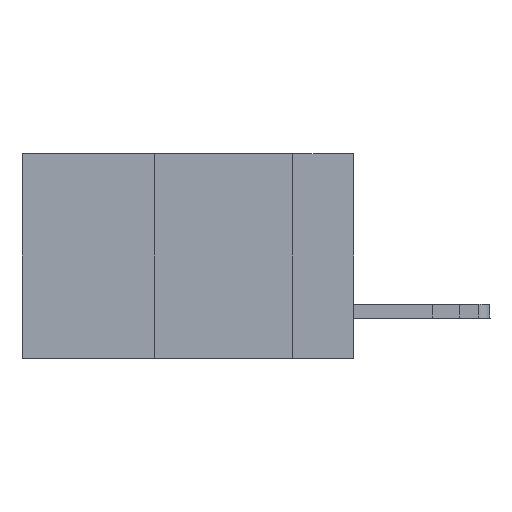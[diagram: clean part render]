
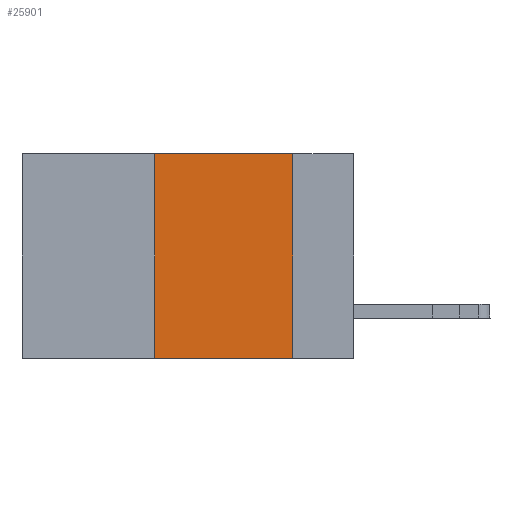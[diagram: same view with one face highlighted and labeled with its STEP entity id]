
A CAD part, left-side view. The second image highlights one B-rep face of the part: STEP entity #25901.
In plain terms, the highlighted planar face has unit normal (-1, 0, 0).
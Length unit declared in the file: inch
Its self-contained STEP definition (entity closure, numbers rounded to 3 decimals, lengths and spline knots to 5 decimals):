
#77 = EDGE_CURVE ( 'NONE', #2742, #160, #29321, .T. ) ;
#160 = VERTEX_POINT ( 'NONE', #16566 ) ;
#452 = VECTOR ( 'NONE', #12100, 39.37008 ) ;
#610 = ORIENTED_EDGE ( 'NONE', *, *, #16156, .F. ) ;
#1116 = CARTESIAN_POINT ( 'NONE',  ( 0., 0.36, -0.37 ) ) ;
#2742 = VERTEX_POINT ( 'NONE', #4361 ) ;
#3239 = VERTEX_POINT ( 'NONE', #1116 ) ;
#3292 = EDGE_LOOP ( 'NONE', ( #15563, #25573, #610, #14857 ) ) ;
#4238 = PLANE ( 'NONE',  #6633 ) ;
#4361 = CARTESIAN_POINT ( 'NONE',  ( 0., 0.36, 0. ) ) ;
#5701 = DIRECTION ( 'NONE',  ( 0., -1., 0. ) ) ;
#6616 = DIRECTION ( 'NONE',  ( 0., 0., -1. ) ) ;
#6633 = AXIS2_PLACEMENT_3D ( 'NONE', #15881, #20581, #6616 ) ;
#6714 = LINE ( 'NONE', #11904, #452 ) ;
#7095 = DIRECTION ( 'NONE',  ( 0., 0., 1. ) ) ;
#8468 = EDGE_CURVE ( 'NONE', #3239, #19511, #11167, .T. ) ;
#10179 = FACE_OUTER_BOUND ( 'NONE', #3292, .T. ) ;
#10399 = CARTESIAN_POINT ( 'NONE',  ( 0., 0.11, -0.37 ) ) ;
#11167 = LINE ( 'NONE', #24411, #17372 ) ;
#11904 = CARTESIAN_POINT ( 'NONE',  ( 0., 0.11, 0. ) ) ;
#12100 = DIRECTION ( 'NONE',  ( 0., 0., -1. ) ) ;
#14304 = CARTESIAN_POINT ( 'NONE',  ( 0., 0.6, 0. ) ) ;
#14857 = ORIENTED_EDGE ( 'NONE', *, *, #8468, .T. ) ;
#15563 = ORIENTED_EDGE ( 'NONE', *, *, #19978, .F. ) ;
#15881 = CARTESIAN_POINT ( 'NONE',  ( 0., 0.6, 0. ) ) ;
#16156 = EDGE_CURVE ( 'NONE', #3239, #2742, #18986, .T. ) ;
#16566 = CARTESIAN_POINT ( 'NONE',  ( 0., 0.11, 0. ) ) ;
#17372 = VECTOR ( 'NONE', #5701, 39.37008 ) ;
#18269 = VECTOR ( 'NONE', #7095, 39.37008 ) ;
#18454 = DIRECTION ( 'NONE',  ( 0., -1., 0. ) ) ;
#18986 = LINE ( 'NONE', #28086, #18269 ) ;
#19511 = VERTEX_POINT ( 'NONE', #10399 ) ;
#19978 = EDGE_CURVE ( 'NONE', #160, #19511, #6714, .T. ) ;
#20581 = DIRECTION ( 'NONE',  ( 1., 0., 0. ) ) ;
#23010 = VECTOR ( 'NONE', #18454, 39.37008 ) ;
#24411 = CARTESIAN_POINT ( 'NONE',  ( 0., 0.6, -0.37 ) ) ;
#25573 = ORIENTED_EDGE ( 'NONE', *, *, #77, .F. ) ;
#25901 = ADVANCED_FACE ( 'NONE', ( #10179 ), #4238, .F. ) ;
#28086 = CARTESIAN_POINT ( 'NONE',  ( 0., 0.36, 0. ) ) ;
#29321 = LINE ( 'NONE', #14304, #23010 ) ;
